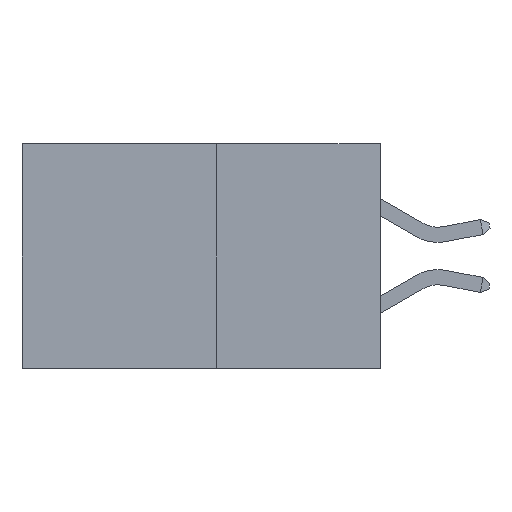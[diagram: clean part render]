
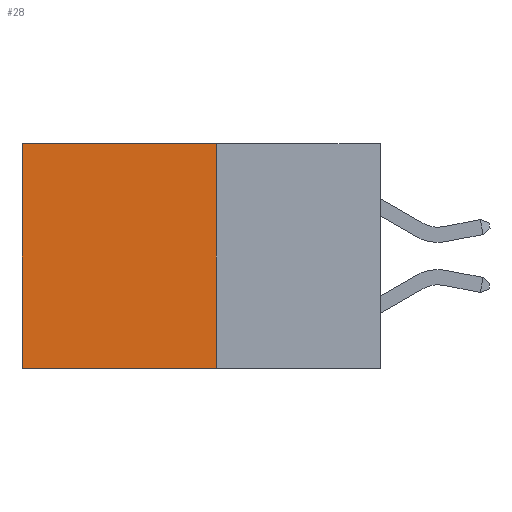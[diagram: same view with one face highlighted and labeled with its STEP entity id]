
A CAD part, left-side view. The second image highlights one B-rep face of the part: STEP entity #28.
In plain terms, the highlighted planar face has unit normal (-1, 0, 0).
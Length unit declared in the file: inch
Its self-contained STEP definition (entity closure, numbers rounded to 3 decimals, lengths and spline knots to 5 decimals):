
#28 = ADVANCED_FACE ( 'NONE', ( #2331 ), #8283, .F. ) ;
#370 = VERTEX_POINT ( 'NONE', #2638 ) ;
#577 = VECTOR ( 'NONE', #7189, 39.37008 ) ;
#737 = DIRECTION ( 'NONE',  ( 0., 0., -1. ) ) ;
#882 = LINE ( 'NONE', #6823, #577 ) ;
#1527 = LINE ( 'NONE', #6115, #6041 ) ;
#2134 = ORIENTED_EDGE ( 'NONE', *, *, #3062, .T. ) ;
#2293 = DIRECTION ( 'NONE',  ( 0., 1., 0. ) ) ;
#2331 = FACE_OUTER_BOUND ( 'NONE', #4112, .T. ) ;
#2638 = CARTESIAN_POINT ( 'NONE',  ( 0.277, 0.59, -0.37 ) ) ;
#2945 = VECTOR ( 'NONE', #4202, 39.37008 ) ;
#3062 = EDGE_CURVE ( 'NONE', #9272, #370, #1527, .T. ) ;
#3320 = CARTESIAN_POINT ( 'NONE',  ( 0.277, 0.27, -0.37 ) ) ;
#3510 = VECTOR ( 'NONE', #2293, 39.37008 ) ;
#4048 = CARTESIAN_POINT ( 'NONE',  ( 0.277, 0.59, 0. ) ) ;
#4112 = EDGE_LOOP ( 'NONE', ( #2134, #4530, #10782, #9141 ) ) ;
#4202 = DIRECTION ( 'NONE',  ( 0., 0., -1. ) ) ;
#4530 = ORIENTED_EDGE ( 'NONE', *, *, #6615, .F. ) ;
#4576 = DIRECTION ( 'NONE',  ( 1., 0., 0. ) ) ;
#4694 = EDGE_CURVE ( 'NONE', #7280, #9272, #882, .T. ) ;
#6041 = VECTOR ( 'NONE', #737, 39.37008 ) ;
#6115 = CARTESIAN_POINT ( 'NONE',  ( 0.277, 0.59, -0.37 ) ) ;
#6225 = LINE ( 'NONE', #6771, #3510 ) ;
#6384 = AXIS2_PLACEMENT_3D ( 'NONE', #7048, #4576, #10422 ) ;
#6615 = EDGE_CURVE ( 'NONE', #9498, #370, #6225, .T. ) ;
#6771 = CARTESIAN_POINT ( 'NONE',  ( 0.277, 0.27, -0.37 ) ) ;
#6777 = EDGE_CURVE ( 'NONE', #7280, #9498, #10018, .T. ) ;
#6823 = CARTESIAN_POINT ( 'NONE',  ( 0.277, 0.27, 0. ) ) ;
#7048 = CARTESIAN_POINT ( 'NONE',  ( 0.277, 0.27, -0.37 ) ) ;
#7189 = DIRECTION ( 'NONE',  ( 0., 1., 0. ) ) ;
#7280 = VERTEX_POINT ( 'NONE', #10107 ) ;
#8283 = PLANE ( 'NONE',  #6384 ) ;
#9141 = ORIENTED_EDGE ( 'NONE', *, *, #4694, .T. ) ;
#9272 = VERTEX_POINT ( 'NONE', #4048 ) ;
#9498 = VERTEX_POINT ( 'NONE', #3320 ) ;
#10018 = LINE ( 'NONE', #10559, #2945 ) ;
#10107 = CARTESIAN_POINT ( 'NONE',  ( 0.277, 0.27, 0. ) ) ;
#10422 = DIRECTION ( 'NONE',  ( 0., 0., -1. ) ) ;
#10559 = CARTESIAN_POINT ( 'NONE',  ( 0.277, 0.27, -0.37 ) ) ;
#10782 = ORIENTED_EDGE ( 'NONE', *, *, #6777, .F. ) ;
